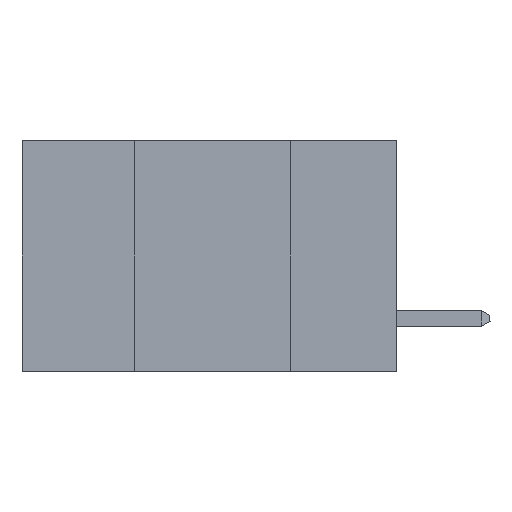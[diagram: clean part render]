
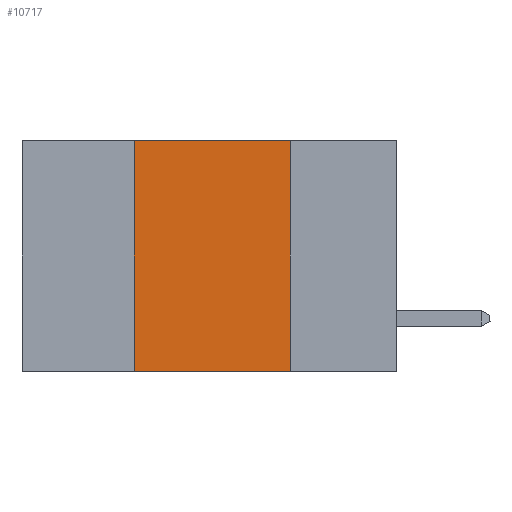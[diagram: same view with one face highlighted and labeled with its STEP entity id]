
A CAD part, left-side view. The second image highlights one B-rep face of the part: STEP entity #10717.
In plain terms, the highlighted planar face has unit normal (-1, 0, 0).
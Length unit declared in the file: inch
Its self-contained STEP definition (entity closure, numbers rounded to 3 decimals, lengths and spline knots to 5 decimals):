
#1422 = PLANE ( 'NONE',  #14174 ) ;
#3521 = DIRECTION ( 'NONE',  ( 0., -1., 0. ) ) ;
#3590 = EDGE_CURVE ( 'NONE', #23416, #17541, #18525, .T. ) ;
#3782 = EDGE_CURVE ( 'NONE', #11710, #15365, #19591, .T. ) ;
#6495 = VECTOR ( 'NONE', #15163, 39.37008 ) ;
#6544 = CARTESIAN_POINT ( 'NONE',  ( 0., 0.17, -0.37 ) ) ;
#7244 = LINE ( 'NONE', #27284, #6495 ) ;
#7677 = VECTOR ( 'NONE', #17253, 39.37008 ) ;
#8551 = DIRECTION ( 'NONE',  ( 1., 0., 0. ) ) ;
#9261 = ORIENTED_EDGE ( 'NONE', *, *, #3782, .T. ) ;
#10541 = VECTOR ( 'NONE', #3521, 39.37008 ) ;
#10717 = ADVANCED_FACE ( 'NONE', ( #11080 ), #1422, .F. ) ;
#10859 = CARTESIAN_POINT ( 'NONE',  ( 0., 0.6, -0.37 ) ) ;
#11080 = FACE_OUTER_BOUND ( 'NONE', #24630, .T. ) ;
#11710 = VERTEX_POINT ( 'NONE', #12485 ) ;
#12485 = CARTESIAN_POINT ( 'NONE',  ( 0., 0.42, -0.37 ) ) ;
#12863 = ORIENTED_EDGE ( 'NONE', *, *, #24045, .F. ) ;
#14174 = AXIS2_PLACEMENT_3D ( 'NONE', #27290, #8551, #24831 ) ;
#14238 = LINE ( 'NONE', #26641, #7677 ) ;
#15163 = DIRECTION ( 'NONE',  ( 0., 0., 1. ) ) ;
#15256 = VECTOR ( 'NONE', #24687, 39.37008 ) ;
#15365 = VERTEX_POINT ( 'NONE', #6544 ) ;
#17253 = DIRECTION ( 'NONE',  ( 0., 0., -1. ) ) ;
#17541 = VERTEX_POINT ( 'NONE', #28506 ) ;
#18525 = LINE ( 'NONE', #29190, #10541 ) ;
#19591 = LINE ( 'NONE', #10859, #15256 ) ;
#21815 = ORIENTED_EDGE ( 'NONE', *, *, #3590, .F. ) ;
#22196 = ORIENTED_EDGE ( 'NONE', *, *, #28335, .F. ) ;
#23416 = VERTEX_POINT ( 'NONE', #27436 ) ;
#24045 = EDGE_CURVE ( 'NONE', #17541, #15365, #14238, .T. ) ;
#24630 = EDGE_LOOP ( 'NONE', ( #12863, #21815, #22196, #9261 ) ) ;
#24687 = DIRECTION ( 'NONE',  ( 0., -1., 0. ) ) ;
#24831 = DIRECTION ( 'NONE',  ( 0., 0., -1. ) ) ;
#26641 = CARTESIAN_POINT ( 'NONE',  ( 0., 0.17, 0. ) ) ;
#27284 = CARTESIAN_POINT ( 'NONE',  ( 0., 0.42, 0. ) ) ;
#27290 = CARTESIAN_POINT ( 'NONE',  ( 0., 0.6, 0. ) ) ;
#27436 = CARTESIAN_POINT ( 'NONE',  ( 0., 0.42, 0. ) ) ;
#28335 = EDGE_CURVE ( 'NONE', #11710, #23416, #7244, .T. ) ;
#28506 = CARTESIAN_POINT ( 'NONE',  ( 0., 0.17, 0. ) ) ;
#29190 = CARTESIAN_POINT ( 'NONE',  ( 0., 0.6, 0. ) ) ;
